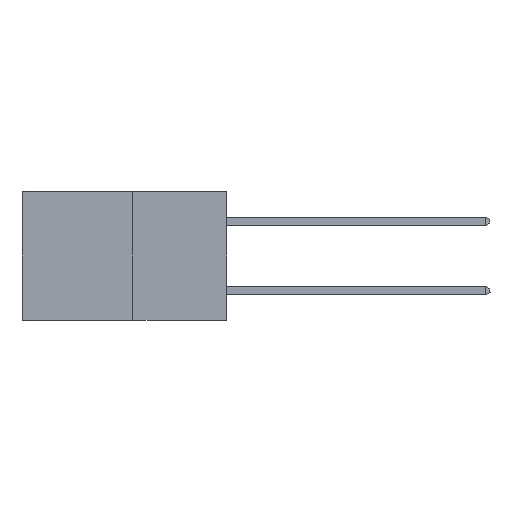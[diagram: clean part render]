
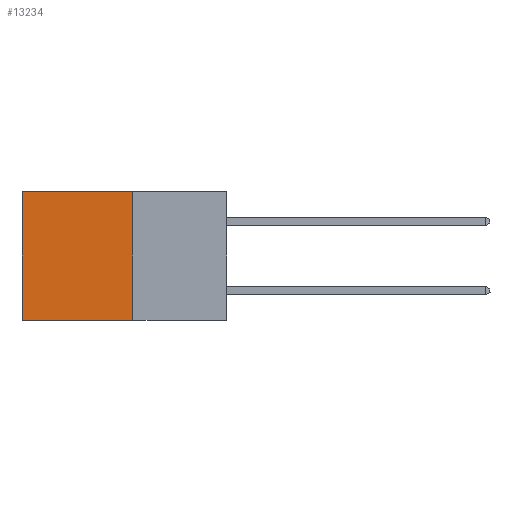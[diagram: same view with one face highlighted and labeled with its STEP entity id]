
A CAD part, left-side view. The second image highlights one B-rep face of the part: STEP entity #13234.
In plain terms, the highlighted planar face has unit normal (-1, 0, 0).
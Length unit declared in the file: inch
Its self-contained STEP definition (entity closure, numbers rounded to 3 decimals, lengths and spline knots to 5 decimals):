
#64 = CARTESIAN_POINT ( 'NONE',  ( 0.277, 0.59, 0. ) ) ;
#939 = VECTOR ( 'NONE', #9394, 39.37008 ) ;
#1447 = DIRECTION ( 'NONE',  ( 1., 0., 0. ) ) ;
#1769 = DIRECTION ( 'NONE',  ( 0., 1., 0. ) ) ;
#1881 = ORIENTED_EDGE ( 'NONE', *, *, #11305, .T. ) ;
#2304 = CARTESIAN_POINT ( 'NONE',  ( 0.277, 0.27, -0.37 ) ) ;
#2335 = CARTESIAN_POINT ( 'NONE',  ( 0.277, 0.27, 0. ) ) ;
#3818 = CARTESIAN_POINT ( 'NONE',  ( 0.277, 0.59, -0.37 ) ) ;
#3820 = VECTOR ( 'NONE', #10610, 39.37008 ) ;
#4178 = CARTESIAN_POINT ( 'NONE',  ( 0.277, 0.27, -0.37 ) ) ;
#4497 = ORIENTED_EDGE ( 'NONE', *, *, #7975, .T. ) ;
#4594 = VERTEX_POINT ( 'NONE', #9697 ) ;
#5030 = DIRECTION ( 'NONE',  ( 0., 0., -1. ) ) ;
#5648 = VERTEX_POINT ( 'NONE', #64 ) ;
#6237 = CARTESIAN_POINT ( 'NONE',  ( 0.277, 0.27, -0.37 ) ) ;
#6637 = EDGE_LOOP ( 'NONE', ( #4497, #12955, #13691, #1881 ) ) ;
#6737 = AXIS2_PLACEMENT_3D ( 'NONE', #6237, #1447, #9748 ) ;
#6771 = CARTESIAN_POINT ( 'NONE',  ( 0.277, 0.59, -0.37 ) ) ;
#7320 = LINE ( 'NONE', #2304, #939 ) ;
#7474 = LINE ( 'NONE', #3818, #7836 ) ;
#7836 = VECTOR ( 'NONE', #5030, 39.37008 ) ;
#7975 = EDGE_CURVE ( 'NONE', #5648, #14213, #7474, .T. ) ;
#8580 = PLANE ( 'NONE',  #6737 ) ;
#9394 = DIRECTION ( 'NONE',  ( 0., 0., -1. ) ) ;
#9697 = CARTESIAN_POINT ( 'NONE',  ( 0.277, 0.27, 0. ) ) ;
#9748 = DIRECTION ( 'NONE',  ( 0., 0., -1. ) ) ;
#10610 = DIRECTION ( 'NONE',  ( 0., 1., 0. ) ) ;
#10976 = FACE_OUTER_BOUND ( 'NONE', #6637, .T. ) ;
#11305 = EDGE_CURVE ( 'NONE', #4594, #5648, #13207, .T. ) ;
#11719 = LINE ( 'NONE', #4178, #14442 ) ;
#12291 = EDGE_CURVE ( 'NONE', #14337, #14213, #11719, .T. ) ;
#12955 = ORIENTED_EDGE ( 'NONE', *, *, #12291, .F. ) ;
#13052 = EDGE_CURVE ( 'NONE', #4594, #14337, #7320, .T. ) ;
#13207 = LINE ( 'NONE', #2335, #3820 ) ;
#13234 = ADVANCED_FACE ( 'NONE', ( #10976 ), #8580, .F. ) ;
#13691 = ORIENTED_EDGE ( 'NONE', *, *, #13052, .F. ) ;
#14213 = VERTEX_POINT ( 'NONE', #6771 ) ;
#14337 = VERTEX_POINT ( 'NONE', #15113 ) ;
#14442 = VECTOR ( 'NONE', #1769, 39.37008 ) ;
#15113 = CARTESIAN_POINT ( 'NONE',  ( 0.277, 0.27, -0.37 ) ) ;
